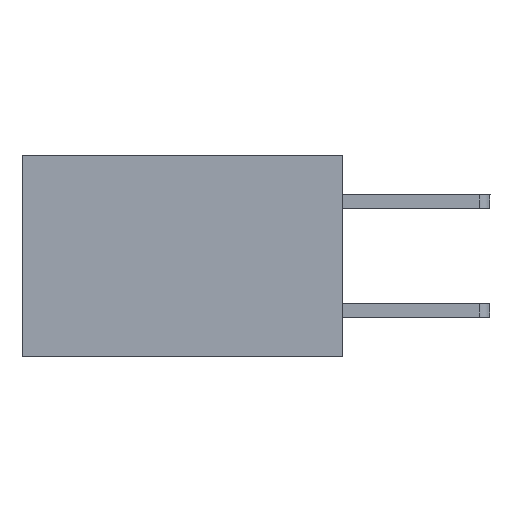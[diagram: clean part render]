
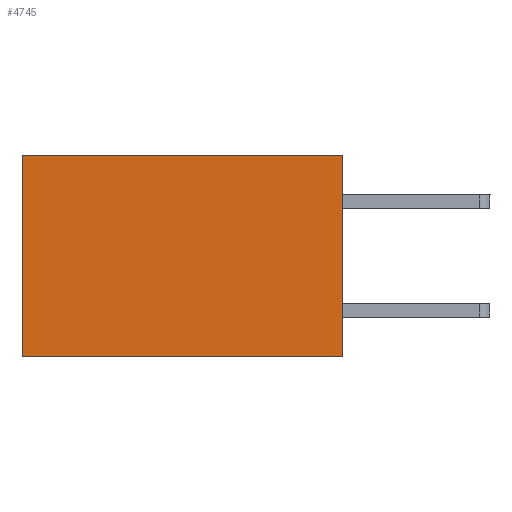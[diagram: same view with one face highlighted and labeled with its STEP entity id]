
A CAD part, left-side view. The second image highlights one B-rep face of the part: STEP entity #4745.
In plain terms, the highlighted planar face has unit normal (-1, 0, 0).
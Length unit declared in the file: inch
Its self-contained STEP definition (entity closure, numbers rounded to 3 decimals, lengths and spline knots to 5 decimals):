
#897 = DIRECTION ( 'NONE',  ( 0., 0., -1. ) ) ;
#914 = DIRECTION ( 'NONE',  ( 0., 0., -1. ) ) ;
#1017 = VERTEX_POINT ( 'NONE', #2994 ) ;
#1027 = EDGE_CURVE ( 'NONE', #9177, #3797, #2889, .T. ) ;
#1277 = LINE ( 'NONE', #4597, #2835 ) ;
#1752 = CARTESIAN_POINT ( 'NONE',  ( 0.277, 0., -0.37 ) ) ;
#2794 = EDGE_LOOP ( 'NONE', ( #9375, #4000, #5921, #11037 ) ) ;
#2835 = VECTOR ( 'NONE', #9785, 39.37008 ) ;
#2889 = LINE ( 'NONE', #9765, #7342 ) ;
#2994 = CARTESIAN_POINT ( 'NONE',  ( 0.277, 0., 0. ) ) ;
#3175 = CARTESIAN_POINT ( 'NONE',  ( 0.277, 0., 0. ) ) ;
#3409 = EDGE_CURVE ( 'NONE', #1017, #9177, #6371, .T. ) ;
#3606 = PLANE ( 'NONE',  #6398 ) ;
#3797 = VERTEX_POINT ( 'NONE', #9928 ) ;
#4000 = ORIENTED_EDGE ( 'NONE', *, *, #7577, .F. ) ;
#4187 = VECTOR ( 'NONE', #897, 39.37008 ) ;
#4597 = CARTESIAN_POINT ( 'NONE',  ( 0.277, 0., -0.37 ) ) ;
#4745 = ADVANCED_FACE ( 'NONE', ( #9471 ), #3606, .F. ) ;
#4985 = VERTEX_POINT ( 'NONE', #9005 ) ;
#5136 = DIRECTION ( 'NONE',  ( 1., 0., 0. ) ) ;
#5921 = ORIENTED_EDGE ( 'NONE', *, *, #9200, .F. ) ;
#6114 = CARTESIAN_POINT ( 'NONE',  ( 0.277, 0.59, 0. ) ) ;
#6371 = LINE ( 'NONE', #3175, #7775 ) ;
#6398 = AXIS2_PLACEMENT_3D ( 'NONE', #1752, #5136, #914 ) ;
#6540 = DIRECTION ( 'NONE',  ( 0., 1., 0. ) ) ;
#7342 = VECTOR ( 'NONE', #9814, 39.37008 ) ;
#7577 = EDGE_CURVE ( 'NONE', #4985, #3797, #1277, .T. ) ;
#7775 = VECTOR ( 'NONE', #6540, 39.37008 ) ;
#8770 = LINE ( 'NONE', #9622, #4187 ) ;
#9005 = CARTESIAN_POINT ( 'NONE',  ( 0.277, 0., -0.37 ) ) ;
#9177 = VERTEX_POINT ( 'NONE', #6114 ) ;
#9200 = EDGE_CURVE ( 'NONE', #1017, #4985, #8770, .T. ) ;
#9375 = ORIENTED_EDGE ( 'NONE', *, *, #1027, .T. ) ;
#9471 = FACE_OUTER_BOUND ( 'NONE', #2794, .T. ) ;
#9622 = CARTESIAN_POINT ( 'NONE',  ( 0.277, 0., -0.37 ) ) ;
#9765 = CARTESIAN_POINT ( 'NONE',  ( 0.277, 0.59, -0.37 ) ) ;
#9785 = DIRECTION ( 'NONE',  ( 0., 1., 0. ) ) ;
#9814 = DIRECTION ( 'NONE',  ( 0., 0., -1. ) ) ;
#9928 = CARTESIAN_POINT ( 'NONE',  ( 0.277, 0.59, -0.37 ) ) ;
#11037 = ORIENTED_EDGE ( 'NONE', *, *, #3409, .T. ) ;
